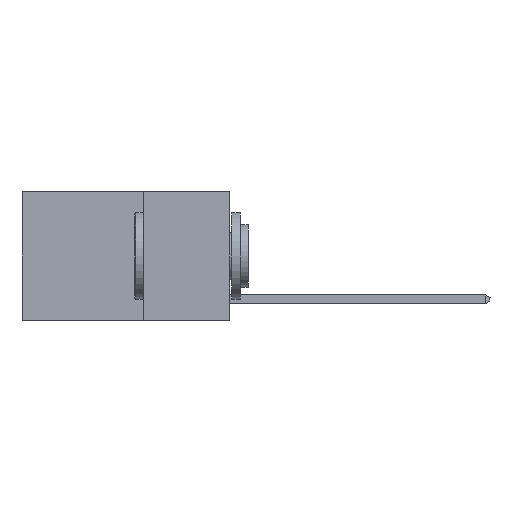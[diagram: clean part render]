
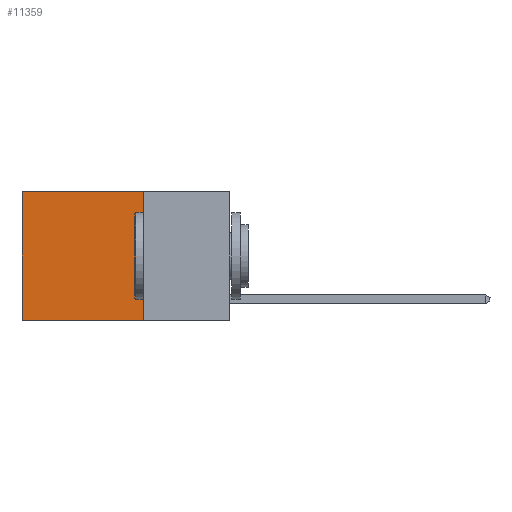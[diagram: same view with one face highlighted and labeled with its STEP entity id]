
A CAD part, left-side view. The second image highlights one B-rep face of the part: STEP entity #11359.
In plain terms, the highlighted planar face has unit normal (-1, 0, 0).
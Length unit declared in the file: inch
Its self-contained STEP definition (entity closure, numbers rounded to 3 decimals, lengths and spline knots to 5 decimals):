
#73 = DIRECTION ( 'NONE',  ( 0., 0., -1. ) ) ;
#288 = EDGE_CURVE ( 'NONE', #4504, #6086, #12355, .T. ) ;
#442 = DIRECTION ( 'NONE',  ( 0., 1., 0. ) ) ;
#539 = CARTESIAN_POINT ( 'NONE',  ( 0.2625, 0.6, 0. ) ) ;
#1267 = CARTESIAN_POINT ( 'NONE',  ( 0.2625, 0.25, -0.37 ) ) ;
#1493 = VECTOR ( 'NONE', #73, 39.37008 ) ;
#1663 = AXIS2_PLACEMENT_3D ( 'NONE', #3043, #4077, #11283 ) ;
#1855 = VECTOR ( 'NONE', #442, 39.37008 ) ;
#1878 = FACE_OUTER_BOUND ( 'NONE', #6344, .T. ) ;
#2343 = DIRECTION ( 'NONE',  ( 0., 0., -1. ) ) ;
#3043 = CARTESIAN_POINT ( 'NONE',  ( 0.2625, 0.25, 0. ) ) ;
#3650 = VECTOR ( 'NONE', #11913, 39.37008 ) ;
#4077 = DIRECTION ( 'NONE',  ( 1., 0., 0. ) ) ;
#4504 = VERTEX_POINT ( 'NONE', #11962 ) ;
#5115 = CARTESIAN_POINT ( 'NONE',  ( 0.2625, 0.25, 0. ) ) ;
#6086 = VERTEX_POINT ( 'NONE', #1267 ) ;
#6344 = EDGE_LOOP ( 'NONE', ( #8892, #9444, #9133, #9534 ) ) ;
#6423 = CARTESIAN_POINT ( 'NONE',  ( 0.2625, 0.6, -0.37 ) ) ;
#7549 = VERTEX_POINT ( 'NONE', #6423 ) ;
#8101 = EDGE_CURVE ( 'NONE', #8943, #7549, #12468, .T. ) ;
#8680 = CARTESIAN_POINT ( 'NONE',  ( 0.2625, 0.25, 0. ) ) ;
#8892 = ORIENTED_EDGE ( 'NONE', *, *, #8101, .T. ) ;
#8943 = VERTEX_POINT ( 'NONE', #539 ) ;
#9126 = LINE ( 'NONE', #10911, #3650 ) ;
#9133 = ORIENTED_EDGE ( 'NONE', *, *, #288, .F. ) ;
#9444 = ORIENTED_EDGE ( 'NONE', *, *, #12930, .F. ) ;
#9510 = CARTESIAN_POINT ( 'NONE',  ( 0.2625, 0.6, 0. ) ) ;
#9534 = ORIENTED_EDGE ( 'NONE', *, *, #12747, .T. ) ;
#9848 = VECTOR ( 'NONE', #2343, 39.37008 ) ;
#10187 = PLANE ( 'NONE',  #1663 ) ;
#10911 = CARTESIAN_POINT ( 'NONE',  ( 0.2625, 0.25, -0.37 ) ) ;
#11283 = DIRECTION ( 'NONE',  ( 0., 0., -1. ) ) ;
#11359 = ADVANCED_FACE ( 'NONE', ( #1878 ), #10187, .F. ) ;
#11913 = DIRECTION ( 'NONE',  ( 0., 1., 0. ) ) ;
#11962 = CARTESIAN_POINT ( 'NONE',  ( 0.2625, 0.25, 0. ) ) ;
#12355 = LINE ( 'NONE', #5115, #1493 ) ;
#12468 = LINE ( 'NONE', #9510, #9848 ) ;
#12747 = EDGE_CURVE ( 'NONE', #4504, #8943, #12972, .T. ) ;
#12930 = EDGE_CURVE ( 'NONE', #6086, #7549, #9126, .T. ) ;
#12972 = LINE ( 'NONE', #8680, #1855 ) ;
